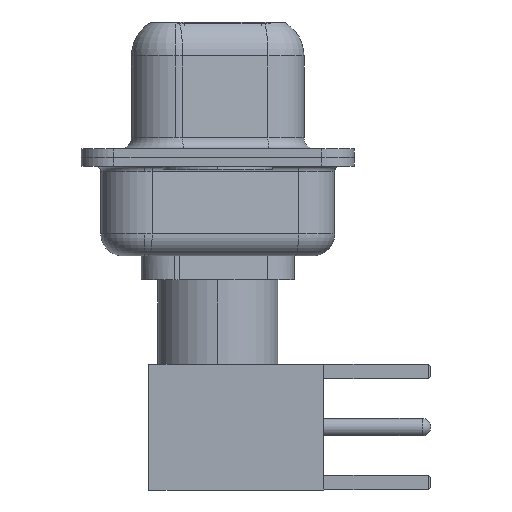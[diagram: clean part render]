
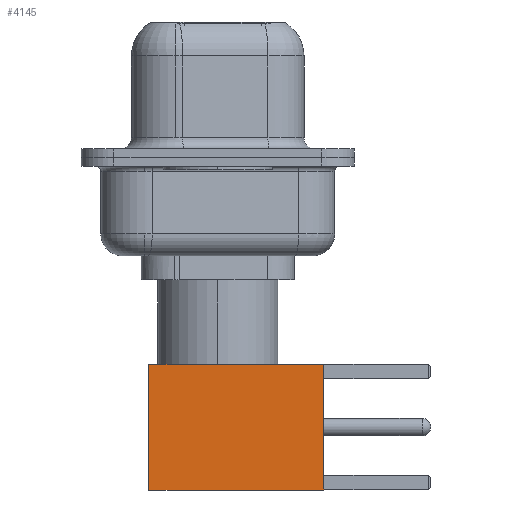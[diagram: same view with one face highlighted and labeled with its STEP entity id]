
A CAD part, left-side view. The second image highlights one B-rep face of the part: STEP entity #4145.
In plain terms, the highlighted face is planar.
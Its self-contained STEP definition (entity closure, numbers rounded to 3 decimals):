
#73 = FACE_OUTER_BOUND ( 'NONE', #3887, .T. ) ;
#498 = DIRECTION ( 'NONE',  ( -1., 0., 0. ) ) ;
#504 = CARTESIAN_POINT ( 'NONE',  ( -2.875, 2.875, 8. ) ) ;
#622 = VERTEX_POINT ( 'NONE', #504 ) ;
#635 = CARTESIAN_POINT ( 'NONE',  ( 0., 2.875, 8. ) ) ;
#830 = VECTOR ( 'NONE', #11334, 1000. ) ;
#1265 = DIRECTION ( 'NONE',  ( 0., 0., 1. ) ) ;
#2000 = ORIENTED_EDGE ( 'NONE', *, *, #8055, .F. ) ;
#2314 = PLANE ( 'NONE',  #12192 ) ;
#2335 = ORIENTED_EDGE ( 'NONE', *, *, #10616, .T. ) ;
#3051 = CARTESIAN_POINT ( 'NONE',  ( 2.875, 2.875, 0. ) ) ;
#3096 = CARTESIAN_POINT ( 'NONE',  ( 0., 2.875, 0. ) ) ;
#3887 = EDGE_LOOP ( 'NONE', ( #11190, #2335, #13380, #2000 ) ) ;
#4145 = ADVANCED_FACE ( 'NONE', ( #73 ), #2314, .T. ) ;
#4467 = EDGE_CURVE ( 'NONE', #622, #13346, #6053, .T. ) ;
#5227 = LINE ( 'NONE', #5540, #9610 ) ;
#5540 = CARTESIAN_POINT ( 'NONE',  ( 2.875, 2.875, 0. ) ) ;
#6053 = LINE ( 'NONE', #10081, #830 ) ;
#6064 = CARTESIAN_POINT ( 'NONE',  ( -2.875, 2.875, 0. ) ) ;
#6561 = CARTESIAN_POINT ( 'NONE',  ( 2.875, 2.875, 0. ) ) ;
#7160 = VECTOR ( 'NONE', #498, 1000. ) ;
#7675 = CARTESIAN_POINT ( 'NONE',  ( 2.875, 2.875, 8. ) ) ;
#7824 = VECTOR ( 'NONE', #8504, 1000. ) ;
#8055 = EDGE_CURVE ( 'NONE', #13222, #622, #8073, .T. ) ;
#8073 = LINE ( 'NONE', #635, #7160 ) ;
#8504 = DIRECTION ( 'NONE',  ( -1., 0., 0. ) ) ;
#8714 = DIRECTION ( 'NONE',  ( 0., 0., -1. ) ) ;
#9610 = VECTOR ( 'NONE', #8714, 1000. ) ;
#10081 = CARTESIAN_POINT ( 'NONE',  ( -2.875, 2.875, 0. ) ) ;
#10538 = LINE ( 'NONE', #3096, #7824 ) ;
#10616 = EDGE_CURVE ( 'NONE', #12585, #13346, #10538, .T. ) ;
#10770 = EDGE_CURVE ( 'NONE', #13222, #12585, #5227, .T. ) ;
#10783 = DIRECTION ( 'NONE',  ( 0., 1., 0. ) ) ;
#11190 = ORIENTED_EDGE ( 'NONE', *, *, #10770, .T. ) ;
#11334 = DIRECTION ( 'NONE',  ( 0., 0., -1. ) ) ;
#12192 = AXIS2_PLACEMENT_3D ( 'NONE', #6561, #10783, #1265 ) ;
#12585 = VERTEX_POINT ( 'NONE', #3051 ) ;
#13222 = VERTEX_POINT ( 'NONE', #7675 ) ;
#13346 = VERTEX_POINT ( 'NONE', #6064 ) ;
#13380 = ORIENTED_EDGE ( 'NONE', *, *, #4467, .F. ) ;
